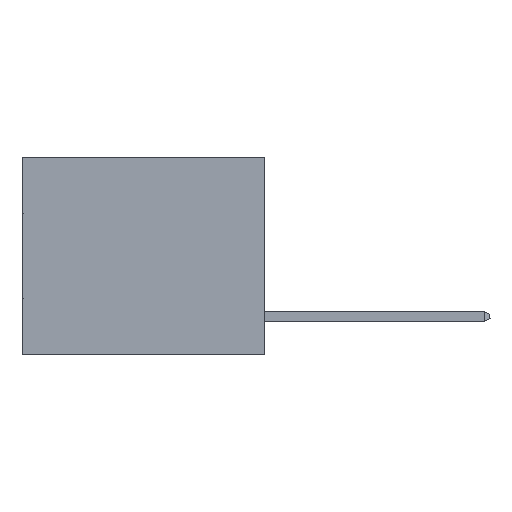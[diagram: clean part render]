
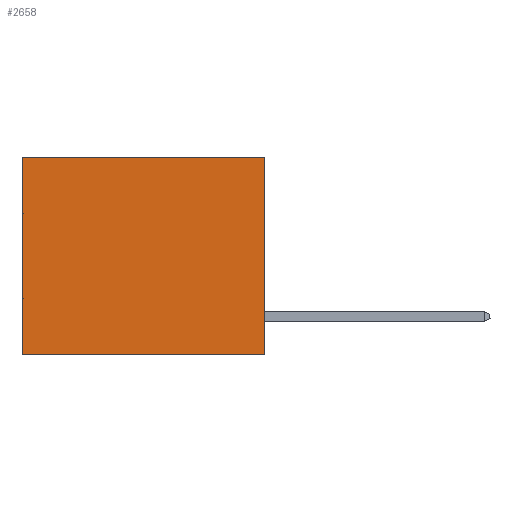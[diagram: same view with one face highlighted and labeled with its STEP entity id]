
A CAD part, left-side view. The second image highlights one B-rep face of the part: STEP entity #2658.
In plain terms, the highlighted planar face has unit normal (-1, 0, 0).
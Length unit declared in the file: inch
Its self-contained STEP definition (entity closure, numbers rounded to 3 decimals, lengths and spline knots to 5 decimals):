
#159 = VECTOR ( 'NONE', #21674, 39.37008 ) ;
#1906 = VECTOR ( 'NONE', #17574, 39.37008 ) ;
#2026 = DIRECTION ( 'NONE',  ( 0., 1., 0. ) ) ;
#2390 = EDGE_LOOP ( 'NONE', ( #2516, #2894, #4279, #19460 ) ) ;
#2516 = ORIENTED_EDGE ( 'NONE', *, *, #16219, .T. ) ;
#2658 = ADVANCED_FACE ( 'NONE', ( #28404 ), #19710, .F. ) ;
#2894 = ORIENTED_EDGE ( 'NONE', *, *, #32673, .F. ) ;
#4279 = ORIENTED_EDGE ( 'NONE', *, *, #10196, .F. ) ;
#6687 = VERTEX_POINT ( 'NONE', #12360 ) ;
#7195 = LINE ( 'NONE', #24695, #159 ) ;
#7964 = DIRECTION ( 'NONE',  ( 0., 0., -1. ) ) ;
#9051 = LINE ( 'NONE', #21373, #29161 ) ;
#9717 = LINE ( 'NONE', #31025, #1906 ) ;
#10196 = EDGE_CURVE ( 'NONE', #24149, #12419, #9051, .T. ) ;
#10275 = CARTESIAN_POINT ( 'NONE',  ( 0.3165, 0., -0.49 ) ) ;
#10734 = VERTEX_POINT ( 'NONE', #20661 ) ;
#12360 = CARTESIAN_POINT ( 'NONE',  ( 0.3165, 0.6, -0.49 ) ) ;
#12419 = VERTEX_POINT ( 'NONE', #28944 ) ;
#14494 = DIRECTION ( 'NONE',  ( 0., 0., -1. ) ) ;
#16219 = EDGE_CURVE ( 'NONE', #10734, #6687, #7195, .T. ) ;
#17574 = DIRECTION ( 'NONE',  ( 0., 1., 0. ) ) ;
#18450 = AXIS2_PLACEMENT_3D ( 'NONE', #24989, #30297, #14494 ) ;
#19460 = ORIENTED_EDGE ( 'NONE', *, *, #23383, .T. ) ;
#19710 = PLANE ( 'NONE',  #18450 ) ;
#20661 = CARTESIAN_POINT ( 'NONE',  ( 0.3165, 0.6, 0. ) ) ;
#21198 = CARTESIAN_POINT ( 'NONE',  ( 0.3165, 0., 0. ) ) ;
#21373 = CARTESIAN_POINT ( 'NONE',  ( 0.3165, 0., -0.49 ) ) ;
#21674 = DIRECTION ( 'NONE',  ( 0., 0., -1. ) ) ;
#22467 = VECTOR ( 'NONE', #2026, 39.37008 ) ;
#23383 = EDGE_CURVE ( 'NONE', #24149, #10734, #9717, .T. ) ;
#24149 = VERTEX_POINT ( 'NONE', #21198 ) ;
#24695 = CARTESIAN_POINT ( 'NONE',  ( 0.3165, 0.6, -0.49 ) ) ;
#24989 = CARTESIAN_POINT ( 'NONE',  ( 0.3165, 0., -0.49 ) ) ;
#28404 = FACE_OUTER_BOUND ( 'NONE', #2390, .T. ) ;
#28944 = CARTESIAN_POINT ( 'NONE',  ( 0.3165, 0., -0.49 ) ) ;
#29161 = VECTOR ( 'NONE', #7964, 39.37008 ) ;
#30297 = DIRECTION ( 'NONE',  ( 1., 0., 0. ) ) ;
#31025 = CARTESIAN_POINT ( 'NONE',  ( 0.3165, 0., 0. ) ) ;
#31171 = LINE ( 'NONE', #10275, #22467 ) ;
#32673 = EDGE_CURVE ( 'NONE', #12419, #6687, #31171, .T. ) ;
